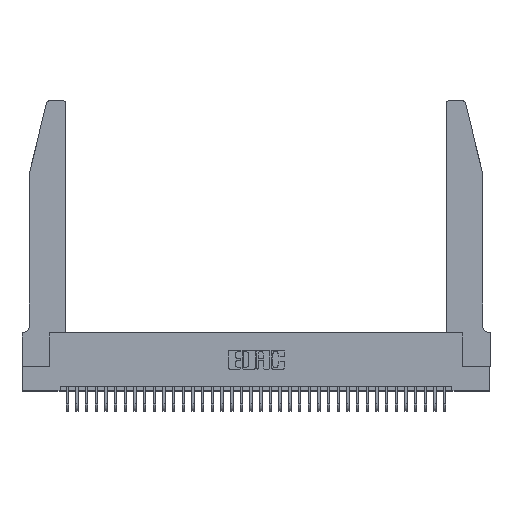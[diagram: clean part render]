
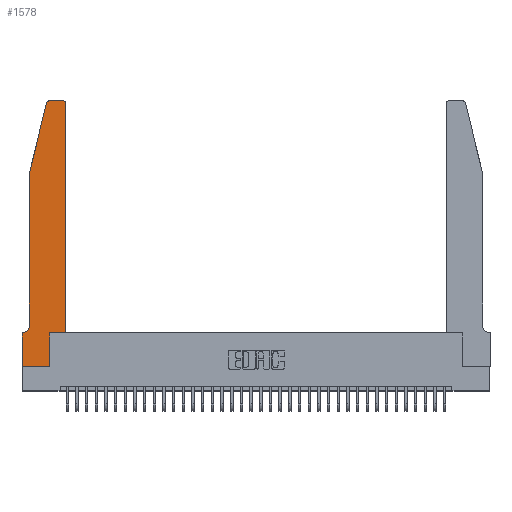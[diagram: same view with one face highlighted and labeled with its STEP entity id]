
A CAD part, top view. The second image highlights one B-rep face of the part: STEP entity #1578.
In plain terms, the highlighted planar face has unit normal (0, 0, 1).
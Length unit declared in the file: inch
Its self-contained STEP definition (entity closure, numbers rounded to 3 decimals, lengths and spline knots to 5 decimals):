
#171 = LINE ( 'NONE', #28826, #29662 ) ;
#226 = VERTEX_POINT ( 'NONE', #21934 ) ;
#1102 = CARTESIAN_POINT ( 'NONE',  ( 0.284, 2.72, 0.37 ) ) ;
#1126 = LINE ( 'NONE', #12984, #34361 ) ;
#1578 = ADVANCED_FACE ( 'NONE', ( #25704 ), #37441, .T. ) ;
#2282 = VERTEX_POINT ( 'NONE', #12386 ) ;
#2503 = CARTESIAN_POINT ( 'NONE',  ( 0.0055, 0.35, 0.37 ) ) ;
#2610 = CARTESIAN_POINT ( 'NONE',  ( 0.0755, 2., 0.37 ) ) ;
#2752 = ORIENTED_EDGE ( 'NONE', *, *, #29801, .T. ) ;
#3566 = AXIS2_PLACEMENT_3D ( 'NONE', #1102, #6858, #30490 ) ;
#3607 = CIRCLE ( 'NONE', #3566, 0.03 ) ;
#3679 = ORIENTED_EDGE ( 'NONE', *, *, #27617, .T. ) ;
#3680 = ORIENTED_EDGE ( 'NONE', *, *, #11420, .T. ) ;
#3682 = ORIENTED_EDGE ( 'NONE', *, *, #20485, .T. ) ;
#3817 = VERTEX_POINT ( 'NONE', #25604 ) ;
#4249 = VERTEX_POINT ( 'NONE', #7435 ) ;
#4478 = EDGE_CURVE ( 'NONE', #7758, #24353, #25504, .T. ) ;
#4703 = EDGE_CURVE ( 'NONE', #28583, #21079, #6978, .T. ) ;
#6180 = AXIS2_PLACEMENT_3D ( 'NONE', #14048, #25691, #37524 ) ;
#6333 = ORIENTED_EDGE ( 'NONE', *, *, #35374, .T. ) ;
#6409 = CIRCLE ( 'NONE', #13978, 0.03 ) ;
#6652 = ORIENTED_EDGE ( 'NONE', *, *, #30684, .T. ) ;
#6858 = DIRECTION ( 'NONE',  ( 0., 0., 1. ) ) ;
#6916 = ORIENTED_EDGE ( 'NONE', *, *, #15081, .T. ) ;
#6978 = LINE ( 'NONE', #9016, #28746 ) ;
#7048 = DIRECTION ( 'NONE',  ( 1., 0., 0. ) ) ;
#7435 = CARTESIAN_POINT ( 'NONE',  ( 0.4205, 2.75, 0.37 ) ) ;
#7474 = ORIENTED_EDGE ( 'NONE', *, *, #16888, .T. ) ;
#7758 = VERTEX_POINT ( 'NONE', #28410 ) ;
#8187 = ORIENTED_EDGE ( 'NONE', *, *, #15074, .T. ) ;
#8196 = DIRECTION ( 'NONE',  ( 0., 1., 0. ) ) ;
#9016 = CARTESIAN_POINT ( 'NONE',  ( 0.4505, 0.35, 0.37 ) ) ;
#9745 = CARTESIAN_POINT ( 'NONE',  ( 0.25487, 2.72718, 0.37 ) ) ;
#10868 = CARTESIAN_POINT ( 'NONE',  ( 0., 0., 0.37 ) ) ;
#11002 = CARTESIAN_POINT ( 'NONE',  ( 0.2865, 0.35, 0.37 ) ) ;
#11420 = EDGE_CURVE ( 'NONE', #3817, #28583, #1126, .T. ) ;
#12169 = LINE ( 'NONE', #17480, #37072 ) ;
#12386 = CARTESIAN_POINT ( 'NONE',  ( 0., 0., 0.37 ) ) ;
#12984 = CARTESIAN_POINT ( 'NONE',  ( 0.4505, 0.35, 0.37 ) ) ;
#13117 = DIRECTION ( 'NONE',  ( 0., 0., 1. ) ) ;
#13978 = AXIS2_PLACEMENT_3D ( 'NONE', #29327, #13117, #7048 ) ;
#14048 = CARTESIAN_POINT ( 'NONE',  ( 0., 0.35, 0.37 ) ) ;
#14239 = DIRECTION ( 'NONE',  ( 0., -1., 0. ) ) ;
#15074 = EDGE_CURVE ( 'NONE', #15603, #3817, #31964, .T. ) ;
#15081 = EDGE_CURVE ( 'NONE', #37606, #7758, #171, .T. ) ;
#15201 = EDGE_LOOP ( 'NONE', ( #2752, #3679, #6916, #18858, #6652, #23917, #6333, #7474, #8187, #3680, #35244, #3682 ) ) ;
#15263 = DIRECTION ( 'NONE',  ( -1., 0., 0. ) ) ;
#15264 = LINE ( 'NONE', #31786, #22665 ) ;
#15336 = VECTOR ( 'NONE', #26180, 39.37008 ) ;
#15603 = VERTEX_POINT ( 'NONE', #23112 ) ;
#15609 = VECTOR ( 'NONE', #23365, 39.37008 ) ;
#16888 = EDGE_CURVE ( 'NONE', #2282, #15603, #25818, .T. ) ;
#17480 = CARTESIAN_POINT ( 'NONE',  ( 0.2605, 2.75, 0.37 ) ) ;
#18657 = DIRECTION ( 'NONE',  ( 1., 0., 0. ) ) ;
#18858 = ORIENTED_EDGE ( 'NONE', *, *, #4478, .T. ) ;
#19967 = CARTESIAN_POINT ( 'NONE',  ( 0.284, 2.75, 0.37 ) ) ;
#20485 = EDGE_CURVE ( 'NONE', #21079, #4249, #6409, .T. ) ;
#20854 = VECTOR ( 'NONE', #8196, 39.37008 ) ;
#21079 = VERTEX_POINT ( 'NONE', #34744 ) ;
#21182 = DIRECTION ( 'NONE',  ( 0., 0., -1. ) ) ;
#21934 = CARTESIAN_POINT ( 'NONE',  ( 0., 0.35, 0.37 ) ) ;
#22665 = VECTOR ( 'NONE', #14239, 39.37008 ) ;
#23112 = CARTESIAN_POINT ( 'NONE',  ( 0.2865, 0., 0.37 ) ) ;
#23365 = DIRECTION ( 'NONE',  ( 1., 0., 0. ) ) ;
#23917 = ORIENTED_EDGE ( 'NONE', *, *, #29847, .T. ) ;
#24353 = VERTEX_POINT ( 'NONE', #26400 ) ;
#25384 = LINE ( 'NONE', #27123, #36826 ) ;
#25504 = LINE ( 'NONE', #2610, #15336 ) ;
#25568 = CIRCLE ( 'NONE', #28314, 0.07 ) ;
#25604 = CARTESIAN_POINT ( 'NONE',  ( 0.2865, 0.35, 0.37 ) ) ;
#25691 = DIRECTION ( 'NONE',  ( 0., 0., 1. ) ) ;
#25704 = FACE_OUTER_BOUND ( 'NONE', #15201, .T. ) ;
#25818 = LINE ( 'NONE', #10868, #15609 ) ;
#25979 = DIRECTION ( 'NONE',  ( -0.239, -0.971, 0. ) ) ;
#26180 = DIRECTION ( 'NONE',  ( 0., -1., 0. ) ) ;
#26400 = CARTESIAN_POINT ( 'NONE',  ( 0.0755, 0.42, 0.37 ) ) ;
#27123 = CARTESIAN_POINT ( 'NONE',  ( 0.0755, 0.35, 0.37 ) ) ;
#27250 = DIRECTION ( 'NONE',  ( -1., 0., 0. ) ) ;
#27617 = EDGE_CURVE ( 'NONE', #29061, #37606, #3607, .T. ) ;
#28314 = AXIS2_PLACEMENT_3D ( 'NONE', #35989, #21182, #15263 ) ;
#28410 = CARTESIAN_POINT ( 'NONE',  ( 0.0755, 2., 0.37 ) ) ;
#28583 = VERTEX_POINT ( 'NONE', #34733 ) ;
#28746 = VECTOR ( 'NONE', #35544, 39.37008 ) ;
#28826 = CARTESIAN_POINT ( 'NONE',  ( 0.0755, 2., 0.37 ) ) ;
#29061 = VERTEX_POINT ( 'NONE', #19967 ) ;
#29327 = CARTESIAN_POINT ( 'NONE',  ( 0.4205, 2.72, 0.37 ) ) ;
#29662 = VECTOR ( 'NONE', #25979, 39.37008 ) ;
#29801 = EDGE_CURVE ( 'NONE', #4249, #29061, #12169, .T. ) ;
#29847 = EDGE_CURVE ( 'NONE', #34126, #226, #25384, .T. ) ;
#30490 = DIRECTION ( 'NONE',  ( 1., 0., 0. ) ) ;
#30684 = EDGE_CURVE ( 'NONE', #24353, #34126, #25568, .T. ) ;
#31786 = CARTESIAN_POINT ( 'NONE',  ( 0., 0., 0.37 ) ) ;
#31964 = LINE ( 'NONE', #11002, #20854 ) ;
#34126 = VERTEX_POINT ( 'NONE', #2503 ) ;
#34361 = VECTOR ( 'NONE', #18657, 39.37008 ) ;
#34733 = CARTESIAN_POINT ( 'NONE',  ( 0.4505, 0.35, 0.37 ) ) ;
#34744 = CARTESIAN_POINT ( 'NONE',  ( 0.4505, 2.72, 0.37 ) ) ;
#35155 = DIRECTION ( 'NONE',  ( -1., 0., 0. ) ) ;
#35244 = ORIENTED_EDGE ( 'NONE', *, *, #4703, .T. ) ;
#35374 = EDGE_CURVE ( 'NONE', #226, #2282, #15264, .T. ) ;
#35544 = DIRECTION ( 'NONE',  ( 0., 1., 0. ) ) ;
#35989 = CARTESIAN_POINT ( 'NONE',  ( 0.0055, 0.42, 0.37 ) ) ;
#36826 = VECTOR ( 'NONE', #27250, 39.37008 ) ;
#37072 = VECTOR ( 'NONE', #35155, 39.37008 ) ;
#37441 = PLANE ( 'NONE',  #6180 ) ;
#37524 = DIRECTION ( 'NONE',  ( 1., 0., 0. ) ) ;
#37606 = VERTEX_POINT ( 'NONE', #9745 ) ;
